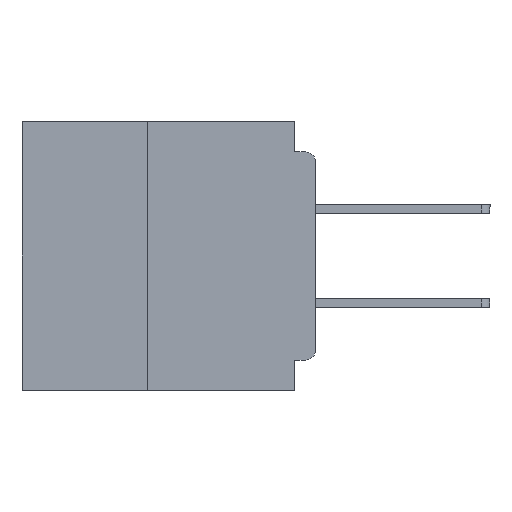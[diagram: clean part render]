
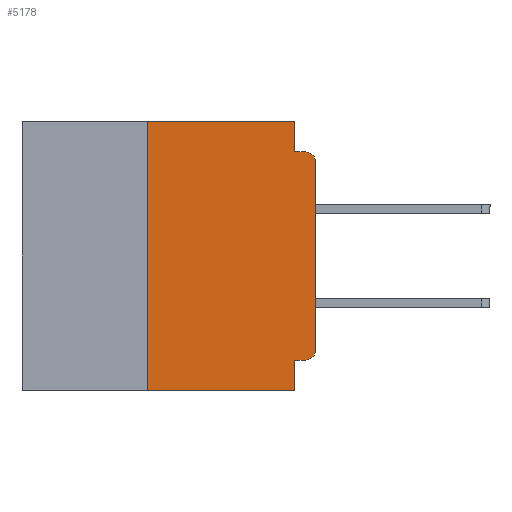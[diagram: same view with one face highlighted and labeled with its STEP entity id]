
A CAD part, left-side view. The second image highlights one B-rep face of the part: STEP entity #5178.
In plain terms, the highlighted planar face has unit normal (-1, 0, 0).
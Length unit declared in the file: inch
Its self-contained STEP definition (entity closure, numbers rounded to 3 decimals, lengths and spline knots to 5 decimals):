
#156 = LINE ( 'NONE', #18087, #44734 ) ;
#681 = ORIENTED_EDGE ( 'NONE', *, *, #36535, .T. ) ;
#701 = DIRECTION ( 'NONE',  ( 0., 0., -1. ) ) ;
#708 = LINE ( 'NONE', #36553, #45234 ) ;
#1524 = CARTESIAN_POINT ( 'NONE',  ( 0., 0.031, -0.4 ) ) ;
#1717 = LINE ( 'NONE', #2093, #10056 ) ;
#2056 = LINE ( 'NONE', #14204, #33522 ) ;
#2093 = CARTESIAN_POINT ( 'NONE',  ( 0., 0.437, 0. ) ) ;
#2119 = ORIENTED_EDGE ( 'NONE', *, *, #35883, .F. ) ;
#2139 = ORIENTED_EDGE ( 'NONE', *, *, #33338, .T. ) ;
#3085 = DIRECTION ( 'NONE',  ( -1., 0., 0. ) ) ;
#3111 = VERTEX_POINT ( 'NONE', #12025 ) ;
#4121 = LINE ( 'NONE', #29391, #32265 ) ;
#5025 = LINE ( 'NONE', #17258, #22723 ) ;
#5178 = ADVANCED_FACE ( 'NONE', ( #41536 ), #39376, .F. ) ;
#6354 = LINE ( 'NONE', #13598, #33381 ) ;
#8232 = EDGE_CURVE ( 'NONE', #3111, #21668, #1717, .T. ) ;
#9812 = EDGE_CURVE ( 'NONE', #24221, #36810, #2056, .T. ) ;
#10056 = VECTOR ( 'NONE', #23307, 39.37008 ) ;
#10909 = ORIENTED_EDGE ( 'NONE', *, *, #19556, .T. ) ;
#11844 = DIRECTION ( 'NONE',  ( 0., 0., 1. ) ) ;
#11851 = DIRECTION ( 'NONE',  ( 0., 0., -1. ) ) ;
#11863 = LINE ( 'NONE', #33441, #29481 ) ;
#12025 = CARTESIAN_POINT ( 'NONE',  ( 0., 0.25, 0. ) ) ;
#13315 = AXIS2_PLACEMENT_3D ( 'NONE', #24290, #3085, #27826 ) ;
#13373 = CARTESIAN_POINT ( 'NONE',  ( 0., 0.031, -0.045 ) ) ;
#13598 = CARTESIAN_POINT ( 'NONE',  ( 0., 0.437, -0.4 ) ) ;
#13969 = CARTESIAN_POINT ( 'NONE',  ( 0., 0., -0.06 ) ) ;
#14204 = CARTESIAN_POINT ( 'NONE',  ( 0., 0., -0.355 ) ) ;
#14251 = CARTESIAN_POINT ( 'NONE',  ( 0., 0., -0.34 ) ) ;
#14265 = CIRCLE ( 'NONE', #31199, 0.015 ) ;
#15061 = ORIENTED_EDGE ( 'NONE', *, *, #27903, .F. ) ;
#15574 = ORIENTED_EDGE ( 'NONE', *, *, #29472, .F. ) ;
#17258 = CARTESIAN_POINT ( 'NONE',  ( 0., 0., -0.045 ) ) ;
#17796 = CARTESIAN_POINT ( 'NONE',  ( 0., 0.25, -0.4 ) ) ;
#18087 = CARTESIAN_POINT ( 'NONE',  ( 0., 0.25, -0.4 ) ) ;
#18199 = DIRECTION ( 'NONE',  ( -1., 0., 0. ) ) ;
#18403 = CARTESIAN_POINT ( 'NONE',  ( 0., 0.437, 0. ) ) ;
#19556 = EDGE_CURVE ( 'NONE', #43743, #26677, #14265, .T. ) ;
#20638 = DIRECTION ( 'NONE',  ( 0., -1., 0. ) ) ;
#20750 = DIRECTION ( 'NONE',  ( 0., -1., 0. ) ) ;
#21610 = DIRECTION ( 'NONE',  ( 0., 0., 1. ) ) ;
#21668 = VERTEX_POINT ( 'NONE', #43421 ) ;
#21931 = DIRECTION ( 'NONE',  ( 1., 0., 0. ) ) ;
#22723 = VECTOR ( 'NONE', #20750, 39.37008 ) ;
#23025 = DIRECTION ( 'NONE',  ( 0., 0., -1. ) ) ;
#23251 = CARTESIAN_POINT ( 'NONE',  ( 0., 0.015, -0.355 ) ) ;
#23307 = DIRECTION ( 'NONE',  ( 0., -1., 0. ) ) ;
#24221 = VERTEX_POINT ( 'NONE', #23251 ) ;
#24290 = CARTESIAN_POINT ( 'NONE',  ( 0., 0.015, -0.34 ) ) ;
#24342 = VERTEX_POINT ( 'NONE', #13373 ) ;
#26677 = VERTEX_POINT ( 'NONE', #35474 ) ;
#27353 = VERTEX_POINT ( 'NONE', #17796 ) ;
#27826 = DIRECTION ( 'NONE',  ( 0., 0., -1. ) ) ;
#27903 = EDGE_CURVE ( 'NONE', #21668, #24342, #708, .T. ) ;
#29032 = CARTESIAN_POINT ( 'NONE',  ( 0., 0.031, -0.355 ) ) ;
#29391 = CARTESIAN_POINT ( 'NONE',  ( 0., 0., 0. ) ) ;
#29472 = EDGE_CURVE ( 'NONE', #24342, #26677, #5025, .T. ) ;
#29481 = VECTOR ( 'NONE', #23025, 39.37008 ) ;
#30189 = VERTEX_POINT ( 'NONE', #14251 ) ;
#31199 = AXIS2_PLACEMENT_3D ( 'NONE', #39177, #18199, #42649 ) ;
#31803 = ORIENTED_EDGE ( 'NONE', *, *, #36949, .F. ) ;
#32265 = VECTOR ( 'NONE', #11844, 39.37008 ) ;
#33338 = EDGE_CURVE ( 'NONE', #27353, #42202, #6354, .T. ) ;
#33381 = VECTOR ( 'NONE', #20638, 39.37008 ) ;
#33441 = CARTESIAN_POINT ( 'NONE',  ( 0., 0.031, -0.4 ) ) ;
#33522 = VECTOR ( 'NONE', #38751, 39.37008 ) ;
#35474 = CARTESIAN_POINT ( 'NONE',  ( 0., 0.015, -0.045 ) ) ;
#35833 = AXIS2_PLACEMENT_3D ( 'NONE', #18403, #21931, #701 ) ;
#35883 = EDGE_CURVE ( 'NONE', #27353, #3111, #156, .T. ) ;
#36209 = EDGE_CURVE ( 'NONE', #30189, #43743, #4121, .T. ) ;
#36535 = EDGE_CURVE ( 'NONE', #24221, #30189, #36608, .T. ) ;
#36553 = CARTESIAN_POINT ( 'NONE',  ( 0., 0.031, 0. ) ) ;
#36608 = CIRCLE ( 'NONE', #13315, 0.015 ) ;
#36810 = VERTEX_POINT ( 'NONE', #29032 ) ;
#36949 = EDGE_CURVE ( 'NONE', #36810, #42202, #11863, .T. ) ;
#37529 = ORIENTED_EDGE ( 'NONE', *, *, #8232, .F. ) ;
#38751 = DIRECTION ( 'NONE',  ( 0., 1., 0. ) ) ;
#39177 = CARTESIAN_POINT ( 'NONE',  ( 0., 0.015, -0.06 ) ) ;
#39376 = PLANE ( 'NONE',  #35833 ) ;
#40437 = ORIENTED_EDGE ( 'NONE', *, *, #36209, .T. ) ;
#41536 = FACE_OUTER_BOUND ( 'NONE', #45237, .T. ) ;
#42202 = VERTEX_POINT ( 'NONE', #1524 ) ;
#42649 = DIRECTION ( 'NONE',  ( 0., 0., -1. ) ) ;
#43421 = CARTESIAN_POINT ( 'NONE',  ( 0., 0.031, 0. ) ) ;
#43580 = ORIENTED_EDGE ( 'NONE', *, *, #9812, .F. ) ;
#43743 = VERTEX_POINT ( 'NONE', #13969 ) ;
#44734 = VECTOR ( 'NONE', #21610, 39.37008 ) ;
#45234 = VECTOR ( 'NONE', #11851, 39.37008 ) ;
#45237 = EDGE_LOOP ( 'NONE', ( #40437, #10909, #15574, #15061, #37529, #2119, #2139, #31803, #43580, #681 ) ) ;
